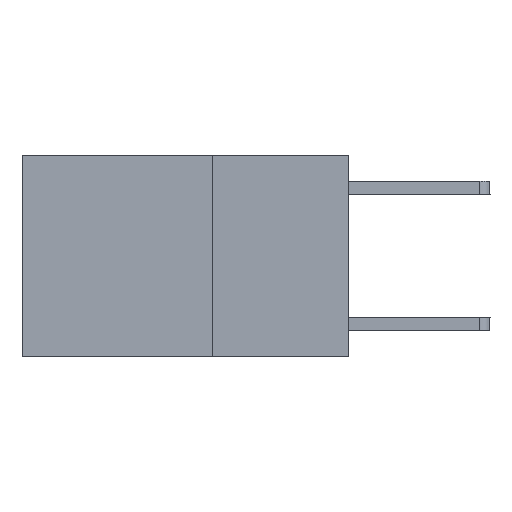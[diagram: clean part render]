
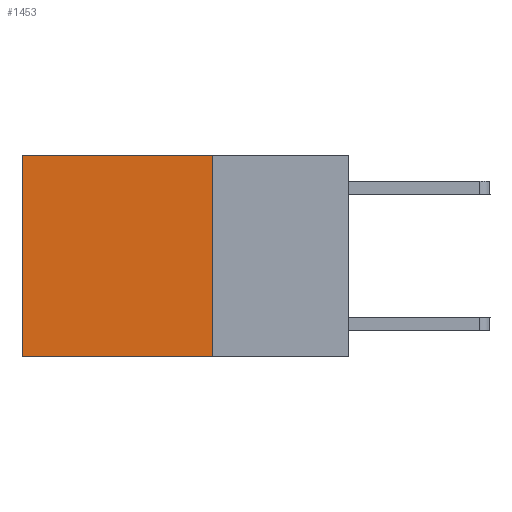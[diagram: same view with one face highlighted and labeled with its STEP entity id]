
A CAD part, left-side view. The second image highlights one B-rep face of the part: STEP entity #1453.
In plain terms, the highlighted planar face has unit normal (-1, 0, 0).
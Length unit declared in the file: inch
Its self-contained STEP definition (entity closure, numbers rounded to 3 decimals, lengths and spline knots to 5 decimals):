
#227 = CARTESIAN_POINT ( 'NONE',  ( 0.2625, 0.6, -0.37 ) ) ;
#290 = CARTESIAN_POINT ( 'NONE',  ( 0.2625, 0.25, 0. ) ) ;
#462 = FACE_OUTER_BOUND ( 'NONE', #3277, .T. ) ;
#844 = LINE ( 'NONE', #9741, #4225 ) ;
#915 = CARTESIAN_POINT ( 'NONE',  ( 0.2625, 0.6, 0. ) ) ;
#1371 = DIRECTION ( 'NONE',  ( 1., 0., 0. ) ) ;
#1391 = VECTOR ( 'NONE', #5875, 39.37008 ) ;
#1453 = ADVANCED_FACE ( 'NONE', ( #462 ), #10923, .F. ) ;
#1617 = DIRECTION ( 'NONE',  ( 0., 0., -1. ) ) ;
#2393 = CARTESIAN_POINT ( 'NONE',  ( 0.2625, 0.25, -0.37 ) ) ;
#2555 = VERTEX_POINT ( 'NONE', #5552 ) ;
#3089 = EDGE_CURVE ( 'NONE', #6794, #2555, #8697, .T. ) ;
#3277 = EDGE_LOOP ( 'NONE', ( #4823, #7769, #11223, #5260 ) ) ;
#3412 = VECTOR ( 'NONE', #4396, 39.37008 ) ;
#3462 = EDGE_CURVE ( 'NONE', #10189, #5909, #10223, .T. ) ;
#3730 = VECTOR ( 'NONE', #7085, 39.37008 ) ;
#4225 = VECTOR ( 'NONE', #8881, 39.37008 ) ;
#4396 = DIRECTION ( 'NONE',  ( 0., 1., 0. ) ) ;
#4699 = CARTESIAN_POINT ( 'NONE',  ( 0.2625, 0.25, 0. ) ) ;
#4823 = ORIENTED_EDGE ( 'NONE', *, *, #10581, .T. ) ;
#5260 = ORIENTED_EDGE ( 'NONE', *, *, #3089, .T. ) ;
#5404 = LINE ( 'NONE', #915, #3730 ) ;
#5552 = CARTESIAN_POINT ( 'NONE',  ( 0.2625, 0.6, 0. ) ) ;
#5875 = DIRECTION ( 'NONE',  ( 0., 1., 0. ) ) ;
#5909 = VERTEX_POINT ( 'NONE', #227 ) ;
#5928 = AXIS2_PLACEMENT_3D ( 'NONE', #290, #1371, #1617 ) ;
#6794 = VERTEX_POINT ( 'NONE', #4699 ) ;
#7085 = DIRECTION ( 'NONE',  ( 0., 0., -1. ) ) ;
#7769 = ORIENTED_EDGE ( 'NONE', *, *, #3462, .F. ) ;
#8697 = LINE ( 'NONE', #8741, #3412 ) ;
#8726 = EDGE_CURVE ( 'NONE', #6794, #10189, #844, .T. ) ;
#8741 = CARTESIAN_POINT ( 'NONE',  ( 0.2625, 0.25, 0. ) ) ;
#8881 = DIRECTION ( 'NONE',  ( 0., 0., -1. ) ) ;
#9741 = CARTESIAN_POINT ( 'NONE',  ( 0.2625, 0.25, 0. ) ) ;
#10189 = VERTEX_POINT ( 'NONE', #10376 ) ;
#10223 = LINE ( 'NONE', #2393, #1391 ) ;
#10376 = CARTESIAN_POINT ( 'NONE',  ( 0.2625, 0.25, -0.37 ) ) ;
#10581 = EDGE_CURVE ( 'NONE', #2555, #5909, #5404, .T. ) ;
#10923 = PLANE ( 'NONE',  #5928 ) ;
#11223 = ORIENTED_EDGE ( 'NONE', *, *, #8726, .F. ) ;
